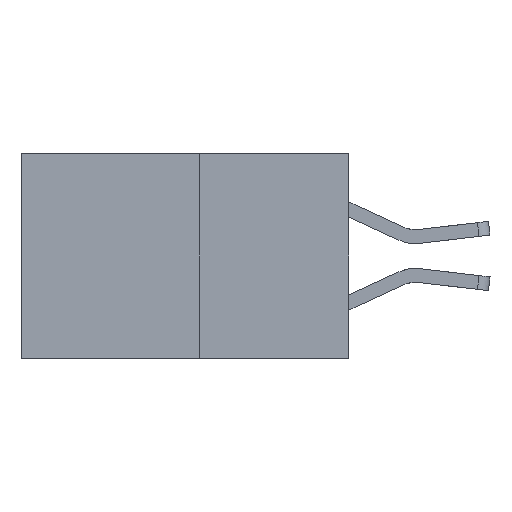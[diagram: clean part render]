
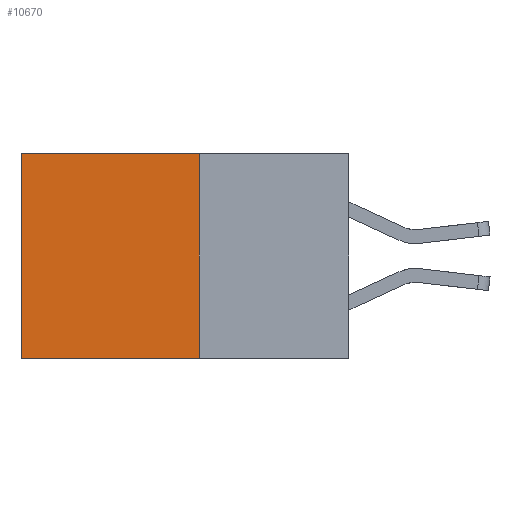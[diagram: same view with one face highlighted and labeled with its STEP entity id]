
A CAD part, left-side view. The second image highlights one B-rep face of the part: STEP entity #10670.
In plain terms, the highlighted planar face has unit normal (-1, 0, 0).
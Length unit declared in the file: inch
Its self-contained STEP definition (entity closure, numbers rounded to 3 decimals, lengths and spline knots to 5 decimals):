
#18 = LINE ( 'NONE', #7865, #2583 ) ;
#781 = DIRECTION ( 'NONE',  ( 1., 0., 0. ) ) ;
#909 = VECTOR ( 'NONE', #2648, 39.37008 ) ;
#1475 = CARTESIAN_POINT ( 'NONE',  ( 0.277, 0.59, -0.37 ) ) ;
#1561 = CARTESIAN_POINT ( 'NONE',  ( 0.277, 0.27, -0.37 ) ) ;
#1830 = PLANE ( 'NONE',  #9864 ) ;
#2180 = EDGE_CURVE ( 'NONE', #8499, #13594, #3620, .T. ) ;
#2583 = VECTOR ( 'NONE', #6798, 39.37008 ) ;
#2648 = DIRECTION ( 'NONE',  ( 0., 1., 0. ) ) ;
#2681 = CARTESIAN_POINT ( 'NONE',  ( 0.277, 0.59, 0. ) ) ;
#2773 = ORIENTED_EDGE ( 'NONE', *, *, #5962, .F. ) ;
#3292 = ORIENTED_EDGE ( 'NONE', *, *, #2180, .T. ) ;
#3464 = VECTOR ( 'NONE', #9161, 39.37008 ) ;
#3611 = DIRECTION ( 'NONE',  ( 0., 0., -1. ) ) ;
#3620 = LINE ( 'NONE', #11448, #3972 ) ;
#3972 = VECTOR ( 'NONE', #3611, 39.37008 ) ;
#4741 = ORIENTED_EDGE ( 'NONE', *, *, #7796, .T. ) ;
#4984 = EDGE_LOOP ( 'NONE', ( #3292, #2773, #5362, #4741 ) ) ;
#5142 = CARTESIAN_POINT ( 'NONE',  ( 0.277, 0.27, -0.37 ) ) ;
#5362 = ORIENTED_EDGE ( 'NONE', *, *, #5960, .F. ) ;
#5960 = EDGE_CURVE ( 'NONE', #10910, #7873, #6369, .T. ) ;
#5962 = EDGE_CURVE ( 'NONE', #7873, #13594, #9242, .T. ) ;
#6369 = LINE ( 'NONE', #13461, #3464 ) ;
#6798 = DIRECTION ( 'NONE',  ( 0., 1., 0. ) ) ;
#6937 = CARTESIAN_POINT ( 'NONE',  ( 0.277, 0.27, -0.37 ) ) ;
#7796 = EDGE_CURVE ( 'NONE', #10910, #8499, #18, .T. ) ;
#7865 = CARTESIAN_POINT ( 'NONE',  ( 0.277, 0.27, 0. ) ) ;
#7873 = VERTEX_POINT ( 'NONE', #6937 ) ;
#8379 = DIRECTION ( 'NONE',  ( 0., 0., -1. ) ) ;
#8499 = VERTEX_POINT ( 'NONE', #2681 ) ;
#8793 = CARTESIAN_POINT ( 'NONE',  ( 0.277, 0.27, 0. ) ) ;
#9161 = DIRECTION ( 'NONE',  ( 0., 0., -1. ) ) ;
#9242 = LINE ( 'NONE', #1561, #909 ) ;
#9864 = AXIS2_PLACEMENT_3D ( 'NONE', #5142, #781, #8379 ) ;
#10249 = FACE_OUTER_BOUND ( 'NONE', #4984, .T. ) ;
#10670 = ADVANCED_FACE ( 'NONE', ( #10249 ), #1830, .F. ) ;
#10910 = VERTEX_POINT ( 'NONE', #8793 ) ;
#11448 = CARTESIAN_POINT ( 'NONE',  ( 0.277, 0.59, -0.37 ) ) ;
#13461 = CARTESIAN_POINT ( 'NONE',  ( 0.277, 0.27, -0.37 ) ) ;
#13594 = VERTEX_POINT ( 'NONE', #1475 ) ;
